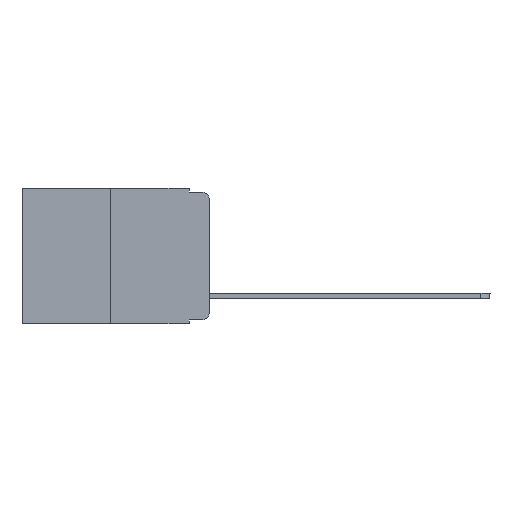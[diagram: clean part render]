
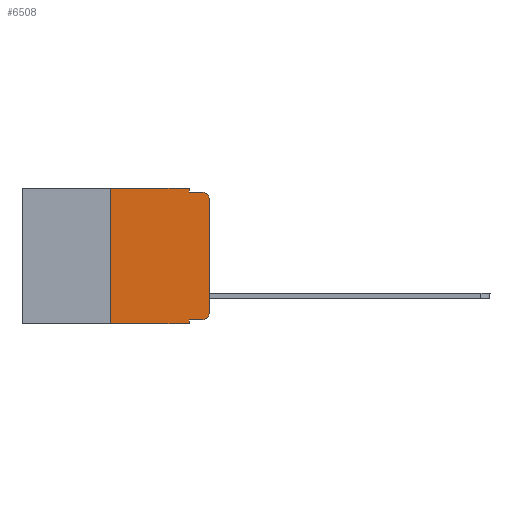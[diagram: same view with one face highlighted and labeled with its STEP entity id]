
A CAD part, left-side view. The second image highlights one B-rep face of the part: STEP entity #6508.
In plain terms, the highlighted planar face has unit normal (-1, 0, 0).
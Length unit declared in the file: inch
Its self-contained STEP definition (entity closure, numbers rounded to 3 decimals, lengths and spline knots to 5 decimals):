
#258 = DIRECTION ( 'NONE',  ( 1., 0., 0. ) ) ;
#449 = CARTESIAN_POINT ( 'NONE',  ( 0., 0.051, 0. ) ) ;
#557 = CIRCLE ( 'NONE', #9304, 0.02 ) ;
#663 = DIRECTION ( 'NONE',  ( 0., 0., 1. ) ) ;
#1275 = CARTESIAN_POINT ( 'NONE',  ( 0., 0.02, -0.03 ) ) ;
#1800 = CARTESIAN_POINT ( 'NONE',  ( 0., 0.051, 0. ) ) ;
#2137 = LINE ( 'NONE', #23459, #20908 ) ;
#2269 = DIRECTION ( 'NONE',  ( 0., -1., 0. ) ) ;
#2565 = CARTESIAN_POINT ( 'NONE',  ( 0., 0., 0. ) ) ;
#3078 = ORIENTED_EDGE ( 'NONE', *, *, #7437, .F. ) ;
#3493 = DIRECTION ( 'NONE',  ( 0., 0., -1. ) ) ;
#3882 = CARTESIAN_POINT ( 'NONE',  ( 0., 0.051, 0. ) ) ;
#4361 = AXIS2_PLACEMENT_3D ( 'NONE', #1275, #13071, #20466 ) ;
#4896 = CARTESIAN_POINT ( 'NONE',  ( 0., 0.473, 0. ) ) ;
#4958 = VERTEX_POINT ( 'NONE', #5792 ) ;
#5073 = AXIS2_PLACEMENT_3D ( 'NONE', #11630, #258, #19374 ) ;
#5265 = LINE ( 'NONE', #2565, #17445 ) ;
#5586 = CARTESIAN_POINT ( 'NONE',  ( 0., 0.051, -0.333 ) ) ;
#5792 = CARTESIAN_POINT ( 'NONE',  ( 0., 0., -0.03 ) ) ;
#5976 = EDGE_CURVE ( 'NONE', #15372, #18574, #18589, .T. ) ;
#6508 = ADVANCED_FACE ( 'NONE', ( #20317 ), #23326, .F. ) ;
#6873 = VERTEX_POINT ( 'NONE', #22414 ) ;
#7201 = EDGE_LOOP ( 'NONE', ( #21961, #17088, #3078, #8641, #19734, #13760, #21969, #11939, #18397, #20289 ) ) ;
#7396 = VERTEX_POINT ( 'NONE', #11273 ) ;
#7437 = EDGE_CURVE ( 'NONE', #12341, #16707, #21446, .T. ) ;
#7670 = CARTESIAN_POINT ( 'NONE',  ( 0., 0., -0.313 ) ) ;
#8078 = VECTOR ( 'NONE', #11901, 39.37008 ) ;
#8641 = ORIENTED_EDGE ( 'NONE', *, *, #24628, .F. ) ;
#8663 = DIRECTION ( 'NONE',  ( -1., 0., 0. ) ) ;
#9304 = AXIS2_PLACEMENT_3D ( 'NONE', #16469, #8663, #10652 ) ;
#9314 = CARTESIAN_POINT ( 'NONE',  ( 0., 0.051, -0.01 ) ) ;
#9347 = EDGE_CURVE ( 'NONE', #11105, #15486, #21966, .T. ) ;
#10605 = CARTESIAN_POINT ( 'NONE',  ( 0., 0.051, -0.333 ) ) ;
#10652 = DIRECTION ( 'NONE',  ( 0., 0., -1. ) ) ;
#10721 = EDGE_CURVE ( 'NONE', #15396, #4958, #5265, .T. ) ;
#11105 = VERTEX_POINT ( 'NONE', #10605 ) ;
#11168 = VECTOR ( 'NONE', #663, 39.37008 ) ;
#11273 = CARTESIAN_POINT ( 'NONE',  ( 0., 0.25, -0.343 ) ) ;
#11630 = CARTESIAN_POINT ( 'NONE',  ( 0., 0.473, 0. ) ) ;
#11901 = DIRECTION ( 'NONE',  ( 0., 0., -1. ) ) ;
#11939 = ORIENTED_EDGE ( 'NONE', *, *, #9347, .F. ) ;
#12341 = VERTEX_POINT ( 'NONE', #16579 ) ;
#13071 = DIRECTION ( 'NONE',  ( -1., 0., 0. ) ) ;
#13531 = VECTOR ( 'NONE', #23884, 39.37008 ) ;
#13760 = ORIENTED_EDGE ( 'NONE', *, *, #22758, .F. ) ;
#13988 = VECTOR ( 'NONE', #3493, 39.37008 ) ;
#14720 = CARTESIAN_POINT ( 'NONE',  ( 0., 0.25, 0. ) ) ;
#15165 = CARTESIAN_POINT ( 'NONE',  ( 0., 0.02, -0.01 ) ) ;
#15208 = LINE ( 'NONE', #5586, #21163 ) ;
#15214 = VECTOR ( 'NONE', #20845, 39.37008 ) ;
#15304 = CARTESIAN_POINT ( 'NONE',  ( 0., 0.051, -0.343 ) ) ;
#15372 = VERTEX_POINT ( 'NONE', #14720 ) ;
#15396 = VERTEX_POINT ( 'NONE', #7670 ) ;
#15486 = VERTEX_POINT ( 'NONE', #15304 ) ;
#16205 = EDGE_CURVE ( 'NONE', #7396, #15486, #2137, .T. ) ;
#16469 = CARTESIAN_POINT ( 'NONE',  ( 0., 0.02, -0.313 ) ) ;
#16579 = CARTESIAN_POINT ( 'NONE',  ( 0., 0.051, -0.01 ) ) ;
#16598 = CIRCLE ( 'NONE', #4361, 0.02 ) ;
#16707 = VERTEX_POINT ( 'NONE', #15165 ) ;
#17088 = ORIENTED_EDGE ( 'NONE', *, *, #20646, .T. ) ;
#17410 = LINE ( 'NONE', #23330, #11168 ) ;
#17445 = VECTOR ( 'NONE', #21529, 39.37008 ) ;
#18397 = ORIENTED_EDGE ( 'NONE', *, *, #23124, .T. ) ;
#18574 = VERTEX_POINT ( 'NONE', #3882 ) ;
#18589 = LINE ( 'NONE', #4896, #13531 ) ;
#18882 = EDGE_CURVE ( 'NONE', #6873, #15396, #557, .T. ) ;
#19374 = DIRECTION ( 'NONE',  ( 0., 0., -1. ) ) ;
#19378 = LINE ( 'NONE', #449, #8078 ) ;
#19734 = ORIENTED_EDGE ( 'NONE', *, *, #5976, .F. ) ;
#20289 = ORIENTED_EDGE ( 'NONE', *, *, #18882, .T. ) ;
#20317 = FACE_OUTER_BOUND ( 'NONE', #7201, .T. ) ;
#20466 = DIRECTION ( 'NONE',  ( 0., 0., -1. ) ) ;
#20646 = EDGE_CURVE ( 'NONE', #4958, #16707, #16598, .T. ) ;
#20720 = DIRECTION ( 'NONE',  ( 0., -1., 0. ) ) ;
#20845 = DIRECTION ( 'NONE',  ( 0., -1., 0. ) ) ;
#20908 = VECTOR ( 'NONE', #2269, 39.37008 ) ;
#21163 = VECTOR ( 'NONE', #20720, 39.37008 ) ;
#21446 = LINE ( 'NONE', #9314, #15214 ) ;
#21529 = DIRECTION ( 'NONE',  ( 0., 0., 1. ) ) ;
#21961 = ORIENTED_EDGE ( 'NONE', *, *, #10721, .T. ) ;
#21966 = LINE ( 'NONE', #1800, #13988 ) ;
#21969 = ORIENTED_EDGE ( 'NONE', *, *, #16205, .T. ) ;
#22414 = CARTESIAN_POINT ( 'NONE',  ( 0., 0.02, -0.333 ) ) ;
#22758 = EDGE_CURVE ( 'NONE', #7396, #15372, #17410, .T. ) ;
#23124 = EDGE_CURVE ( 'NONE', #11105, #6873, #15208, .T. ) ;
#23326 = PLANE ( 'NONE',  #5073 ) ;
#23330 = CARTESIAN_POINT ( 'NONE',  ( 0., 0.25, 0. ) ) ;
#23459 = CARTESIAN_POINT ( 'NONE',  ( 0., 0.473, -0.343 ) ) ;
#23884 = DIRECTION ( 'NONE',  ( 0., -1., 0. ) ) ;
#24628 = EDGE_CURVE ( 'NONE', #18574, #12341, #19378, .T. ) ;
